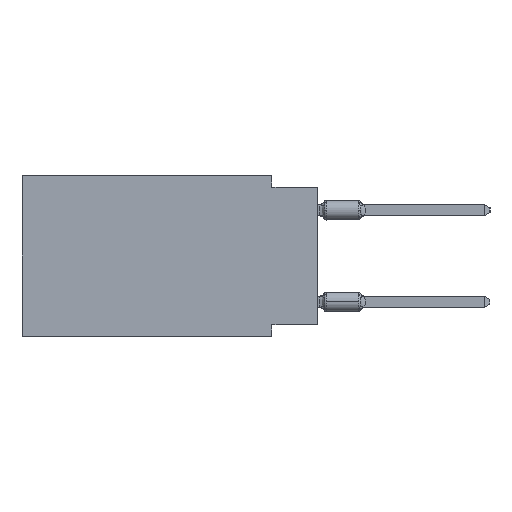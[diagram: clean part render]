
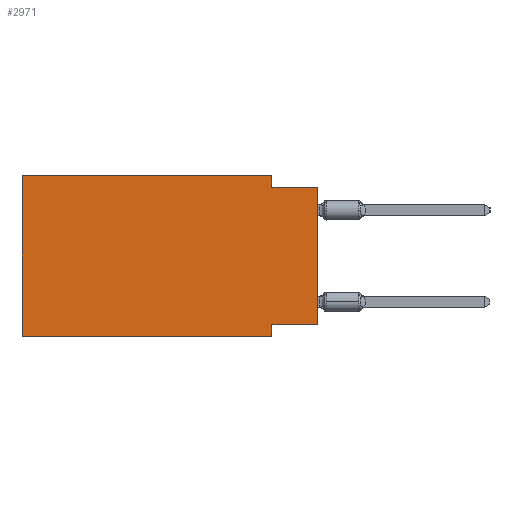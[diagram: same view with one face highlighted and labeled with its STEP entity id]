
A CAD part, left-side view. The second image highlights one B-rep face of the part: STEP entity #2971.
In plain terms, the highlighted planar face has unit normal (-1, 0, 0).
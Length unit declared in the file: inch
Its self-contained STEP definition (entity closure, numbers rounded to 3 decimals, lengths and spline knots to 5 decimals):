
#824 = CARTESIAN_POINT ( 'NONE',  ( 0., 0., -0.325 ) ) ;
#1009 = FACE_OUTER_BOUND ( 'NONE', #30164, .T. ) ;
#1646 = VERTEX_POINT ( 'NONE', #31936 ) ;
#2179 = VECTOR ( 'NONE', #11557, 39.37008 ) ;
#2936 = CARTESIAN_POINT ( 'NONE',  ( 0., 0.645, 0. ) ) ;
#2971 = ADVANCED_FACE ( 'NONE', ( #1009 ), #8590, .F. ) ;
#3296 = LINE ( 'NONE', #45717, #14302 ) ;
#4431 = EDGE_CURVE ( 'NONE', #9984, #47903, #37531, .T. ) ;
#4578 = ORIENTED_EDGE ( 'NONE', *, *, #13857, .F. ) ;
#4855 = CARTESIAN_POINT ( 'NONE',  ( 0., 0.1, 0. ) ) ;
#5933 = CARTESIAN_POINT ( 'NONE',  ( 0., 0.645, -0.35 ) ) ;
#6776 = ORIENTED_EDGE ( 'NONE', *, *, #32766, .F. ) ;
#8034 = VECTOR ( 'NONE', #36367, 39.37008 ) ;
#8590 = PLANE ( 'NONE',  #19029 ) ;
#9331 = EDGE_CURVE ( 'NONE', #9984, #37340, #46155, .T. ) ;
#9984 = VERTEX_POINT ( 'NONE', #5933 ) ;
#11557 = DIRECTION ( 'NONE',  ( 0., 0., 1. ) ) ;
#12214 = VECTOR ( 'NONE', #14912, 39.37008 ) ;
#12670 = VERTEX_POINT ( 'NONE', #47139 ) ;
#12871 = ORIENTED_EDGE ( 'NONE', *, *, #25533, .F. ) ;
#13112 = VERTEX_POINT ( 'NONE', #824 ) ;
#13857 = EDGE_CURVE ( 'NONE', #37340, #12670, #41663, .T. ) ;
#14302 = VECTOR ( 'NONE', #37910, 39.37008 ) ;
#14484 = CARTESIAN_POINT ( 'NONE',  ( 0., 0.1, -0.025 ) ) ;
#14912 = DIRECTION ( 'NONE',  ( 0., -1., 0. ) ) ;
#15432 = CARTESIAN_POINT ( 'NONE',  ( 0., 0.645, 0. ) ) ;
#16431 = DIRECTION ( 'NONE',  ( 0., 0., -1. ) ) ;
#16701 = LINE ( 'NONE', #4855, #28153 ) ;
#18049 = VERTEX_POINT ( 'NONE', #14484 ) ;
#18317 = EDGE_CURVE ( 'NONE', #13112, #1646, #3296, .T. ) ;
#18713 = ORIENTED_EDGE ( 'NONE', *, *, #9331, .F. ) ;
#19029 = AXIS2_PLACEMENT_3D ( 'NONE', #23993, #20226, #16431 ) ;
#19179 = VECTOR ( 'NONE', #45364, 39.37008 ) ;
#19997 = EDGE_CURVE ( 'NONE', #13112, #20383, #36382, .T. ) ;
#20226 = DIRECTION ( 'NONE',  ( 1., 0., 0. ) ) ;
#20383 = VERTEX_POINT ( 'NONE', #44782 ) ;
#20634 = ORIENTED_EDGE ( 'NONE', *, *, #4431, .T. ) ;
#20954 = CARTESIAN_POINT ( 'NONE',  ( 0., 0.1, -0.35 ) ) ;
#21252 = ORIENTED_EDGE ( 'NONE', *, *, #19997, .T. ) ;
#23993 = CARTESIAN_POINT ( 'NONE',  ( 0., 0.645, 0. ) ) ;
#25533 = EDGE_CURVE ( 'NONE', #12670, #18049, #16701, .T. ) ;
#26643 = CARTESIAN_POINT ( 'NONE',  ( 0., 0.1, -0.35 ) ) ;
#27822 = DIRECTION ( 'NONE',  ( 0., 0., -1. ) ) ;
#28153 = VECTOR ( 'NONE', #27822, 39.37008 ) ;
#28255 = ORIENTED_EDGE ( 'NONE', *, *, #18317, .F. ) ;
#30164 = EDGE_LOOP ( 'NONE', ( #21252, #32275, #12871, #4578, #18713, #20634, #6776, #28255 ) ) ;
#31936 = CARTESIAN_POINT ( 'NONE',  ( 0., 0.1, -0.325 ) ) ;
#32275 = ORIENTED_EDGE ( 'NONE', *, *, #34817, .F. ) ;
#32589 = CARTESIAN_POINT ( 'NONE',  ( 0., 0., 0. ) ) ;
#32766 = EDGE_CURVE ( 'NONE', #1646, #47903, #32802, .T. ) ;
#32802 = LINE ( 'NONE', #20954, #8034 ) ;
#33585 = CARTESIAN_POINT ( 'NONE',  ( 0., 0., -0.025 ) ) ;
#34817 = EDGE_CURVE ( 'NONE', #18049, #20383, #48512, .T. ) ;
#34836 = VECTOR ( 'NONE', #40910, 39.37008 ) ;
#36367 = DIRECTION ( 'NONE',  ( 0., 0., -1. ) ) ;
#36382 = LINE ( 'NONE', #32589, #46588 ) ;
#37340 = VERTEX_POINT ( 'NONE', #2936 ) ;
#37531 = LINE ( 'NONE', #37784, #19179 ) ;
#37784 = CARTESIAN_POINT ( 'NONE',  ( 0., 0.645, -0.35 ) ) ;
#37910 = DIRECTION ( 'NONE',  ( 0., 1., 0. ) ) ;
#38309 = CARTESIAN_POINT ( 'NONE',  ( 0., 0.645, 0. ) ) ;
#40910 = DIRECTION ( 'NONE',  ( 0., -1., 0. ) ) ;
#41663 = LINE ( 'NONE', #15432, #12214 ) ;
#44782 = CARTESIAN_POINT ( 'NONE',  ( 0., 0., -0.025 ) ) ;
#45364 = DIRECTION ( 'NONE',  ( 0., -1., 0. ) ) ;
#45717 = CARTESIAN_POINT ( 'NONE',  ( 0., 0., -0.325 ) ) ;
#46155 = LINE ( 'NONE', #38309, #2179 ) ;
#46588 = VECTOR ( 'NONE', #47978, 39.37008 ) ;
#47139 = CARTESIAN_POINT ( 'NONE',  ( 0., 0.1, 0. ) ) ;
#47903 = VERTEX_POINT ( 'NONE', #26643 ) ;
#47978 = DIRECTION ( 'NONE',  ( 0., 0., 1. ) ) ;
#48512 = LINE ( 'NONE', #33585, #34836 ) ;
